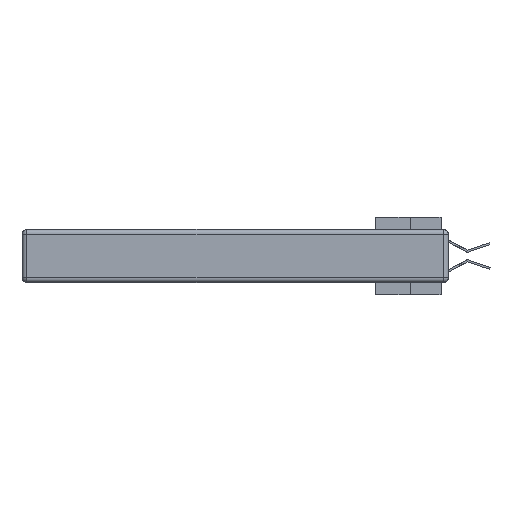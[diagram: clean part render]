
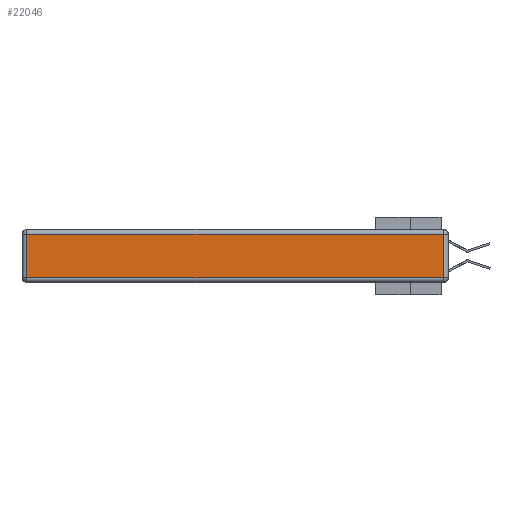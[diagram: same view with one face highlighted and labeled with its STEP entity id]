
A CAD part, left-side view. The second image highlights one B-rep face of the part: STEP entity #22046.
In plain terms, the highlighted planar face has unit normal (-1, 0, 0).
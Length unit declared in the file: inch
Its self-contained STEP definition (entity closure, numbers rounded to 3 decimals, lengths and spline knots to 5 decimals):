
#210 = CARTESIAN_POINT ( 'NONE',  ( 0., 0., -0.313 ) ) ;
#823 = LINE ( 'NONE', #210, #3224 ) ;
#1373 = EDGE_CURVE ( 'NONE', #27481, #3160, #34269, .T. ) ;
#1808 = AXIS2_PLACEMENT_3D ( 'NONE', #11801, #40037, #27258 ) ;
#2974 = DIRECTION ( 'NONE',  ( 0., 1., 0. ) ) ;
#3160 = VERTEX_POINT ( 'NONE', #31716 ) ;
#3224 = VECTOR ( 'NONE', #13345, 39.37008 ) ;
#5933 = CARTESIAN_POINT ( 'NONE',  ( 0., 2.72, -0.343 ) ) ;
#7344 = VERTEX_POINT ( 'NONE', #14627 ) ;
#8864 = DIRECTION ( 'NONE',  ( 0., 0., 1. ) ) ;
#9110 = VECTOR ( 'NONE', #8864, 39.37008 ) ;
#11801 = CARTESIAN_POINT ( 'NONE',  ( 0., 0., -0.343 ) ) ;
#11958 = LINE ( 'NONE', #37105, #9110 ) ;
#13345 = DIRECTION ( 'NONE',  ( 0., -1., 0. ) ) ;
#13836 = EDGE_LOOP ( 'NONE', ( #30554, #39581, #22418, #28662 ) ) ;
#14627 = CARTESIAN_POINT ( 'NONE',  ( 0., 0.03, -0.313 ) ) ;
#15289 = PLANE ( 'NONE',  #1808 ) ;
#15586 = LINE ( 'NONE', #5933, #24348 ) ;
#22046 = ADVANCED_FACE ( 'NONE', ( #37346 ), #15289, .T. ) ;
#22418 = ORIENTED_EDGE ( 'NONE', *, *, #1373, .T. ) ;
#23111 = VECTOR ( 'NONE', #2974, 39.37008 ) ;
#23920 = EDGE_CURVE ( 'NONE', #7344, #27481, #11958, .T. ) ;
#24348 = VECTOR ( 'NONE', #27567, 39.37008 ) ;
#27258 = DIRECTION ( 'NONE',  ( 0., 0., 1. ) ) ;
#27481 = VERTEX_POINT ( 'NONE', #28493 ) ;
#27567 = DIRECTION ( 'NONE',  ( 0., 0., -1. ) ) ;
#28493 = CARTESIAN_POINT ( 'NONE',  ( 0., 0.03, -0.03 ) ) ;
#28662 = ORIENTED_EDGE ( 'NONE', *, *, #34775, .T. ) ;
#30554 = ORIENTED_EDGE ( 'NONE', *, *, #33149, .T. ) ;
#31163 = CARTESIAN_POINT ( 'NONE',  ( 0., 2.75, -0.03 ) ) ;
#31716 = CARTESIAN_POINT ( 'NONE',  ( 0., 2.72, -0.03 ) ) ;
#33128 = CARTESIAN_POINT ( 'NONE',  ( 0., 2.72, -0.313 ) ) ;
#33149 = EDGE_CURVE ( 'NONE', #39822, #7344, #823, .T. ) ;
#34269 = LINE ( 'NONE', #31163, #23111 ) ;
#34775 = EDGE_CURVE ( 'NONE', #3160, #39822, #15586, .T. ) ;
#37105 = CARTESIAN_POINT ( 'NONE',  ( 0., 0.03, -0.343 ) ) ;
#37346 = FACE_OUTER_BOUND ( 'NONE', #13836, .T. ) ;
#39581 = ORIENTED_EDGE ( 'NONE', *, *, #23920, .T. ) ;
#39822 = VERTEX_POINT ( 'NONE', #33128 ) ;
#40037 = DIRECTION ( 'NONE',  ( -1., 0., 0. ) ) ;
